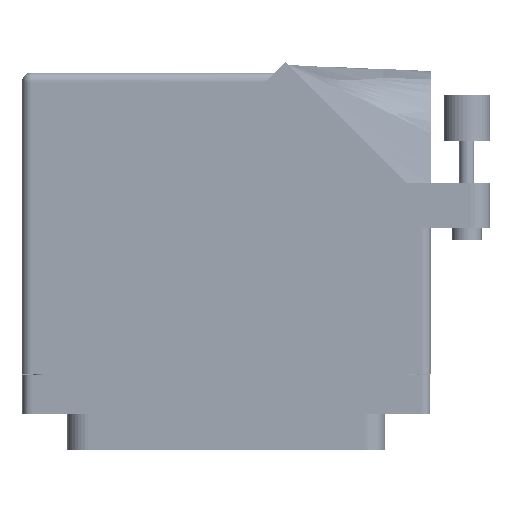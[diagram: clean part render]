
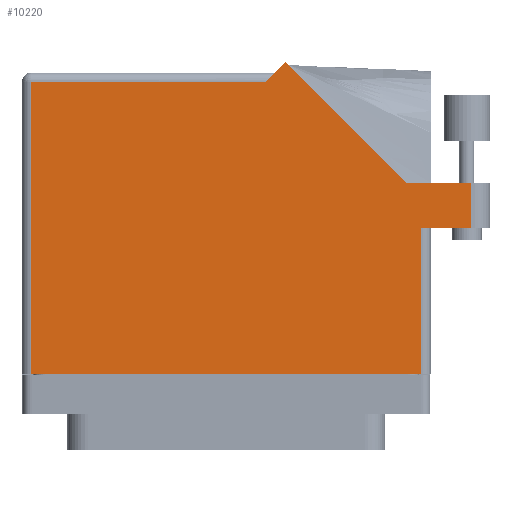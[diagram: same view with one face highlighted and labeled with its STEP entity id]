
A CAD part, front view. The second image highlights one B-rep face of the part: STEP entity #10220.
In plain terms, the highlighted face is planar.
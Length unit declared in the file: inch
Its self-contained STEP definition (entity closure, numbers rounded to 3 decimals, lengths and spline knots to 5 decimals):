
#841 = LINE ( 'NONE', #28398, #55504 ) ;
#3974 = ORIENTED_EDGE ( 'NONE', *, *, #17109, .T. ) ;
#6151 = CARTESIAN_POINT ( 'NONE',  ( -1.3155, -0.1, 0.765 ) ) ;
#6213 = EDGE_CURVE ( 'NONE', #32616, #7881, #52721, .T. ) ;
#6464 = EDGE_CURVE ( 'NONE', #58982, #73051, #83764, .T. ) ;
#6909 = VECTOR ( 'NONE', #21107, 39.37008 ) ;
#7881 = VERTEX_POINT ( 'NONE', #50862 ) ;
#8104 = LINE ( 'NONE', #54698, #25582 ) ;
#8723 = DIRECTION ( 'NONE',  ( 0., 1., 0. ) ) ;
#8971 = FACE_OUTER_BOUND ( 'NONE', #23289, .T. ) ;
#9263 = VERTEX_POINT ( 'NONE', #21978 ) ;
#9389 = VERTEX_POINT ( 'NONE', #15192 ) ;
#10220 = ADVANCED_FACE ( 'NONE', ( #8971 ), #27189, .F. ) ;
#13286 = DIRECTION ( 'NONE',  ( 0., 1., 0. ) ) ;
#14153 = EDGE_CURVE ( 'NONE', #73051, #9389, #841, .T. ) ;
#14460 = DIRECTION ( 'NONE',  ( -0.707, -0.707, 0. ) ) ;
#15010 = ORIENTED_EDGE ( 'NONE', *, *, #14153, .T. ) ;
#15192 = CARTESIAN_POINT ( 'NONE',  ( 1.21192, 1.187, 0.765 ) ) ;
#16187 = CARTESIAN_POINT ( 'NONE',  ( -1.3775, 1.93, 0.765 ) ) ;
#17109 = EDGE_CURVE ( 'NONE', #78446, #55468, #8104, .T. ) ;
#20074 = LINE ( 'NONE', #54874, #67056 ) ;
#20524 = CARTESIAN_POINT ( 'NONE',  ( 1.6525, 1.187, 0.765 ) ) ;
#20785 = ORIENTED_EDGE ( 'NONE', *, *, #6213, .T. ) ;
#21107 = DIRECTION ( 'NONE',  ( -1., 0., 0. ) ) ;
#21851 = CARTESIAN_POINT ( 'NONE',  ( 1.6525, 1.187, 0.765 ) ) ;
#21978 = CARTESIAN_POINT ( 'NONE',  ( -1.3155, 1.868, 0.765 ) ) ;
#23289 = EDGE_LOOP ( 'NONE', ( #28646, #51094, #15010, #57571, #3974, #65758, #87816, #20785, #61858 ) ) ;
#24522 = EDGE_CURVE ( 'NONE', #9389, #78446, #39272, .T. ) ;
#25582 = VECTOR ( 'NONE', #14460, 39.37008 ) ;
#27189 = PLANE ( 'NONE',  #81158 ) ;
#28060 = VECTOR ( 'NONE', #48148, 39.37008 ) ;
#28398 = CARTESIAN_POINT ( 'NONE',  ( 1.7775, 1.187, 0.765 ) ) ;
#28646 = ORIENTED_EDGE ( 'NONE', *, *, #56794, .T. ) ;
#30664 = CARTESIAN_POINT ( 'NONE',  ( 1.3775, 0.88, 0.765 ) ) ;
#32121 = VECTOR ( 'NONE', #88095, 39.37008 ) ;
#32616 = VERTEX_POINT ( 'NONE', #36128 ) ;
#34538 = VECTOR ( 'NONE', #8723, 39.37008 ) ;
#36080 = DIRECTION ( 'NONE',  ( 0., 0., -1. ) ) ;
#36128 = CARTESIAN_POINT ( 'NONE',  ( -1.3155, -0.1, 0.765 ) ) ;
#37042 = VECTOR ( 'NONE', #58243, 39.37008 ) ;
#37448 = LINE ( 'NONE', #30664, #37042 ) ;
#39272 = LINE ( 'NONE', #59640, #32121 ) ;
#42314 = LINE ( 'NONE', #55461, #6909 ) ;
#42399 = EDGE_CURVE ( 'NONE', #55468, #9263, #42314, .T. ) ;
#46590 = CARTESIAN_POINT ( 'NONE',  ( 1.6525, 0.88, 0.765 ) ) ;
#48148 = DIRECTION ( 'NONE',  ( 0., -1., 0. ) ) ;
#50862 = CARTESIAN_POINT ( 'NONE',  ( 1.3155, -0.1, 0.765 ) ) ;
#51094 = ORIENTED_EDGE ( 'NONE', *, *, #6464, .T. ) ;
#52721 = LINE ( 'NONE', #86182, #61691 ) ;
#53175 = DIRECTION ( 'NONE',  ( 1., 0., 0. ) ) ;
#54022 = CARTESIAN_POINT ( 'NONE',  ( 0.2655, 1.868, 0.765 ) ) ;
#54698 = CARTESIAN_POINT ( 'NONE',  ( 0.3275, 1.93, 0.765 ) ) ;
#54874 = CARTESIAN_POINT ( 'NONE',  ( 1.3155, 0.88, 0.765 ) ) ;
#55098 = DIRECTION ( 'NONE',  ( -1., 0., 0. ) ) ;
#55461 = CARTESIAN_POINT ( 'NONE',  ( -1.3775, 1.868, 0.765 ) ) ;
#55468 = VERTEX_POINT ( 'NONE', #54022 ) ;
#55504 = VECTOR ( 'NONE', #55098, 39.37008 ) ;
#56794 = EDGE_CURVE ( 'NONE', #71214, #58982, #37448, .T. ) ;
#57571 = ORIENTED_EDGE ( 'NONE', *, *, #24522, .T. ) ;
#58243 = DIRECTION ( 'NONE',  ( 1., 0., 0. ) ) ;
#58982 = VERTEX_POINT ( 'NONE', #46590 ) ;
#59640 = CARTESIAN_POINT ( 'NONE',  ( 1.21192, 1.187, 0.765 ) ) ;
#61691 = VECTOR ( 'NONE', #53175, 39.37008 ) ;
#61858 = ORIENTED_EDGE ( 'NONE', *, *, #85637, .T. ) ;
#64264 = CARTESIAN_POINT ( 'NONE',  ( 0.39821, 2.00071, 0.765 ) ) ;
#65758 = ORIENTED_EDGE ( 'NONE', *, *, #42399, .T. ) ;
#67056 = VECTOR ( 'NONE', #13286, 39.37008 ) ;
#71214 = VERTEX_POINT ( 'NONE', #73075 ) ;
#73051 = VERTEX_POINT ( 'NONE', #20524 ) ;
#73075 = CARTESIAN_POINT ( 'NONE',  ( 1.3155, 0.88, 0.765 ) ) ;
#78446 = VERTEX_POINT ( 'NONE', #64264 ) ;
#81158 = AXIS2_PLACEMENT_3D ( 'NONE', #16187, #36080, #89103 ) ;
#83764 = LINE ( 'NONE', #21851, #34538 ) ;
#85637 = EDGE_CURVE ( 'NONE', #7881, #71214, #20074, .T. ) ;
#86182 = CARTESIAN_POINT ( 'NONE',  ( -1.3775, -0.1, 0.765 ) ) ;
#87500 = LINE ( 'NONE', #6151, #28060 ) ;
#87816 = ORIENTED_EDGE ( 'NONE', *, *, #89124, .T. ) ;
#88095 = DIRECTION ( 'NONE',  ( -0.707, 0.707, 0. ) ) ;
#89103 = DIRECTION ( 'NONE',  ( -1., 0., 0. ) ) ;
#89124 = EDGE_CURVE ( 'NONE', #9263, #32616, #87500, .T. ) ;
